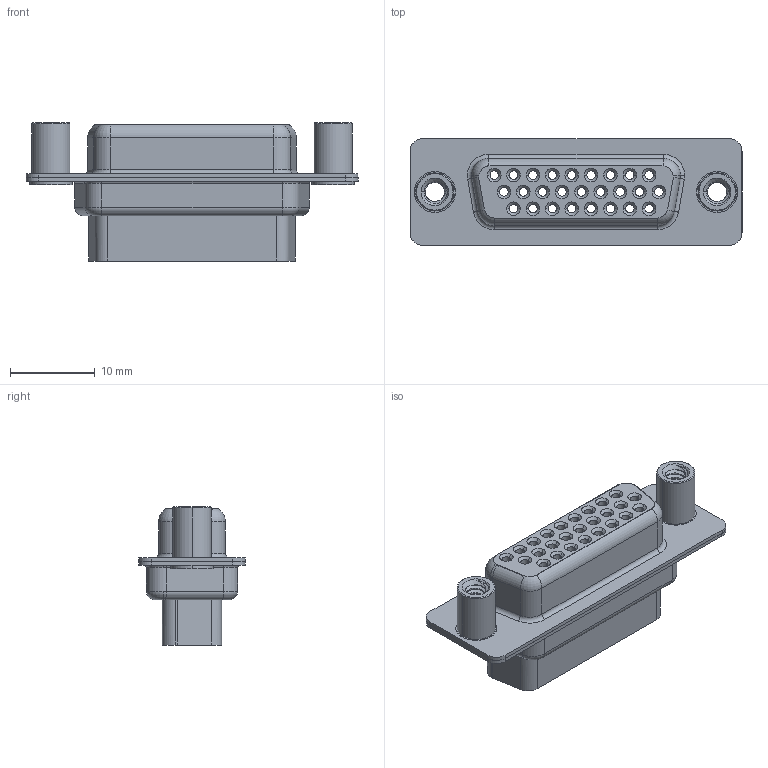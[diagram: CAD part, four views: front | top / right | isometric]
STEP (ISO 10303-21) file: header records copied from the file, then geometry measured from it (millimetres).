
FILE_DESCRIPTION (( 'STEP AP203' ), '1' );
FILE_NAME ('638-026-010-248.STEP', '2020-07-18T16:38:54', ( '' ), ( '' ), 'SwSTEP 2.0', 'SolidWorks 2020', '' );
FILE_SCHEMA (( 'CONFIG_CONTROL_DESIGN' ));
Length unit declared in the file: millimetre
Products named in the file (5): 638-026-010-248; 638 Shell Rear_26 Contacts; 638 Shell Front_26 Contacts; 638 Housing_26 Contacts HP; 638 4-40 Threaded Standoff
Assembly tree (5 placements, depth 2):
  638-026-010-248
    638 Housing_26 Contacts HP
    638 Shell Front_26 Contacts
    638 Shell Rear_26 Contacts
    638 4-40 Threaded Standoff  x2
Bounding box: 39.19 x 12.6 x 16.3 mm (x, y, z)
Volume: 2440.6 mm3; surface area: 6632.2 mm2
Topology: 5 solids, 5 shells, 651 faces, 1505 edges, 955 vertices
Faces by surface type: cylinder 373, plane 147, cone 68, torus 57, bspline 6
Entity records: 19518 total; most frequent: CARTESIAN_POINT 4800, DIRECTION 3242, ORIENTED_EDGE 2756, EDGE_CURVE 1378, AXIS2_PLACEMENT_3D 1359, VERTEX_POINT 873, EDGE_LOOP 755, CIRCLE 753
